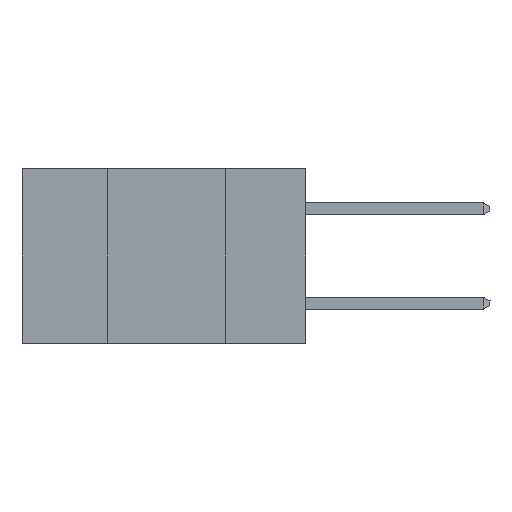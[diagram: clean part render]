
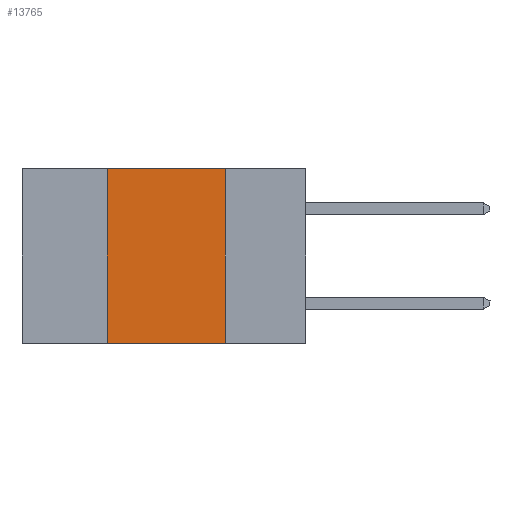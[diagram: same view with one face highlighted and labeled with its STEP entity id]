
A CAD part, left-side view. The second image highlights one B-rep face of the part: STEP entity #13765.
In plain terms, the highlighted planar face has unit normal (-1, 0, 0).
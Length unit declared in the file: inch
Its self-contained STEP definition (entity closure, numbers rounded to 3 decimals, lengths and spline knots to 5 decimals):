
#32 = EDGE_CURVE ( 'NONE', #8875, #2436, #10042, .T. ) ;
#1527 = CARTESIAN_POINT ( 'NONE',  ( 0., 0.17, -0.37 ) ) ;
#1618 = CARTESIAN_POINT ( 'NONE',  ( 0., 0.42, -0.37 ) ) ;
#1778 = CARTESIAN_POINT ( 'NONE',  ( 0., 0.17, 0. ) ) ;
#2308 = VECTOR ( 'NONE', #16041, 39.37008 ) ;
#2436 = VERTEX_POINT ( 'NONE', #1778 ) ;
#2540 = FACE_OUTER_BOUND ( 'NONE', #5997, .T. ) ;
#2610 = ORIENTED_EDGE ( 'NONE', *, *, #11871, .F. ) ;
#3169 = DIRECTION ( 'NONE',  ( 0., -1., 0. ) ) ;
#4044 = DIRECTION ( 'NONE',  ( 0., 0., -1. ) ) ;
#5576 = EDGE_CURVE ( 'NONE', #16141, #20649, #14639, .T. ) ;
#5997 = EDGE_LOOP ( 'NONE', ( #6055, #12936, #2610, #7927 ) ) ;
#6055 = ORIENTED_EDGE ( 'NONE', *, *, #18410, .F. ) ;
#6899 = VECTOR ( 'NONE', #3169, 39.37008 ) ;
#7927 = ORIENTED_EDGE ( 'NONE', *, *, #5576, .T. ) ;
#8875 = VERTEX_POINT ( 'NONE', #11048 ) ;
#8924 = AXIS2_PLACEMENT_3D ( 'NONE', #12121, #16073, #20922 ) ;
#10042 = LINE ( 'NONE', #19800, #6899 ) ;
#10989 = CARTESIAN_POINT ( 'NONE',  ( 0., 0.6, -0.37 ) ) ;
#11048 = CARTESIAN_POINT ( 'NONE',  ( 0., 0.42, 0. ) ) ;
#11362 = LINE ( 'NONE', #12724, #21342 ) ;
#11871 = EDGE_CURVE ( 'NONE', #16141, #8875, #19135, .T. ) ;
#12121 = CARTESIAN_POINT ( 'NONE',  ( 0., 0.6, 0. ) ) ;
#12724 = CARTESIAN_POINT ( 'NONE',  ( 0., 0.17, 0. ) ) ;
#12936 = ORIENTED_EDGE ( 'NONE', *, *, #32, .F. ) ;
#13765 = ADVANCED_FACE ( 'NONE', ( #2540 ), #20613, .F. ) ;
#14639 = LINE ( 'NONE', #10989, #2308 ) ;
#16041 = DIRECTION ( 'NONE',  ( 0., -1., 0. ) ) ;
#16073 = DIRECTION ( 'NONE',  ( 1., 0., 0. ) ) ;
#16141 = VERTEX_POINT ( 'NONE', #1618 ) ;
#16232 = DIRECTION ( 'NONE',  ( 0., 0., 1. ) ) ;
#16362 = CARTESIAN_POINT ( 'NONE',  ( 0., 0.42, 0. ) ) ;
#18410 = EDGE_CURVE ( 'NONE', #2436, #20649, #11362, .T. ) ;
#19135 = LINE ( 'NONE', #16362, #20411 ) ;
#19800 = CARTESIAN_POINT ( 'NONE',  ( 0., 0.6, 0. ) ) ;
#20411 = VECTOR ( 'NONE', #16232, 39.37008 ) ;
#20613 = PLANE ( 'NONE',  #8924 ) ;
#20649 = VERTEX_POINT ( 'NONE', #1527 ) ;
#20922 = DIRECTION ( 'NONE',  ( 0., 0., -1. ) ) ;
#21342 = VECTOR ( 'NONE', #4044, 39.37008 ) ;
